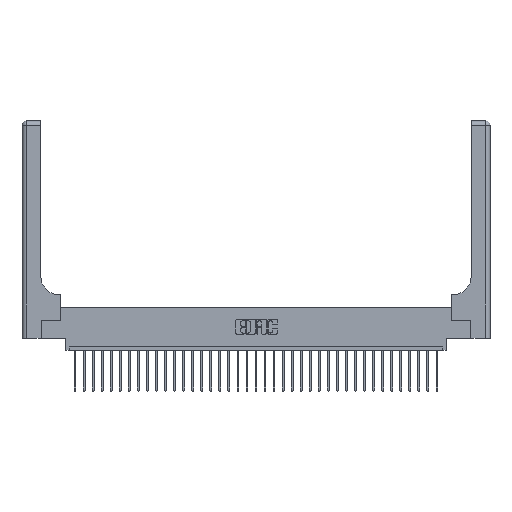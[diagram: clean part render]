
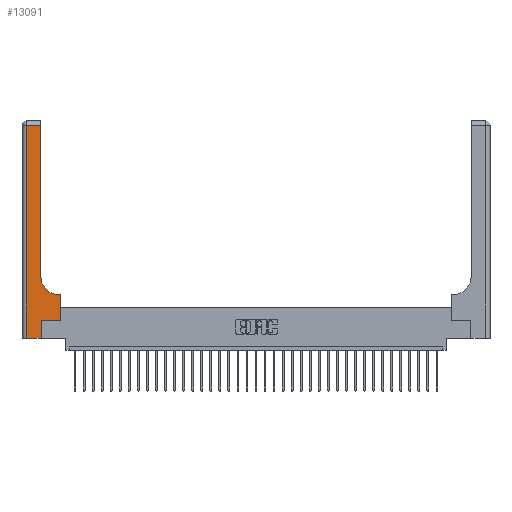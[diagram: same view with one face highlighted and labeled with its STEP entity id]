
A CAD part, top view. The second image highlights one B-rep face of the part: STEP entity #13091.
In plain terms, the highlighted planar face has unit normal (0, 0, 1).
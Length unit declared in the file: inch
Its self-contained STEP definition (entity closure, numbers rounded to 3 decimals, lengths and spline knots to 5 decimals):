
#125 = DIRECTION ( 'NONE',  ( 1., 0., 0. ) ) ;
#1809 = CARTESIAN_POINT ( 'NONE',  ( 0.06, 0., 0.37 ) ) ;
#1960 = DIRECTION ( 'NONE',  ( -1., 0., 0. ) ) ;
#2320 = CARTESIAN_POINT ( 'NONE',  ( 0.51, 0.85, 0.37 ) ) ;
#2383 = CARTESIAN_POINT ( 'NONE',  ( 0.528, 0.25, 0.37 ) ) ;
#2593 = VECTOR ( 'NONE', #26936, 39.37008 ) ;
#3012 = FACE_OUTER_BOUND ( 'NONE', #13031, .T. ) ;
#3409 = EDGE_CURVE ( 'NONE', #23320, #7445, #30415, .T. ) ;
#4195 = LINE ( 'NONE', #17015, #16470 ) ;
#4759 = DIRECTION ( 'NONE',  ( 0., 0., -1. ) ) ;
#5008 = AXIS2_PLACEMENT_3D ( 'NONE', #2320, #4759, #28682 ) ;
#5239 = CARTESIAN_POINT ( 'NONE',  ( 0.528, 0.6, 0.37 ) ) ;
#5479 = EDGE_CURVE ( 'NONE', #10834, #18629, #26133, .T. ) ;
#5733 = CARTESIAN_POINT ( 'NONE',  ( 0.265, 0.25, 0.37 ) ) ;
#6533 = VERTEX_POINT ( 'NONE', #14862 ) ;
#6943 = VECTOR ( 'NONE', #17289, 39.37008 ) ;
#7005 = PLANE ( 'NONE',  #17234 ) ;
#7445 = VERTEX_POINT ( 'NONE', #5239 ) ;
#8553 = CARTESIAN_POINT ( 'NONE',  ( 0., 2.94, 0.37 ) ) ;
#9556 = VECTOR ( 'NONE', #28426, 39.37008 ) ;
#9853 = CARTESIAN_POINT ( 'NONE',  ( 0.26, 0.85, 0.37 ) ) ;
#10433 = CARTESIAN_POINT ( 'NONE',  ( 0.265, 0., 0.37 ) ) ;
#10435 = CARTESIAN_POINT ( 'NONE',  ( 0.265, 0.25, 0.37 ) ) ;
#10453 = LINE ( 'NONE', #10433, #2593 ) ;
#10834 = VERTEX_POINT ( 'NONE', #20953 ) ;
#11054 = VECTOR ( 'NONE', #26046, 39.37008 ) ;
#11936 = CARTESIAN_POINT ( 'NONE',  ( 0., 3., 0.37 ) ) ;
#11959 = CARTESIAN_POINT ( 'NONE',  ( 0.26, 3., 0.37 ) ) ;
#11973 = EDGE_CURVE ( 'NONE', #17200, #23320, #24290, .T. ) ;
#12100 = ORIENTED_EDGE ( 'NONE', *, *, #3409, .T. ) ;
#12642 = CARTESIAN_POINT ( 'NONE',  ( 0.06, 3., 0.37 ) ) ;
#13011 = ORIENTED_EDGE ( 'NONE', *, *, #28578, .T. ) ;
#13031 = EDGE_LOOP ( 'NONE', ( #13040, #22648, #26580, #20272, #13011, #15381, #12100, #23800, #23835 ) ) ;
#13040 = ORIENTED_EDGE ( 'NONE', *, *, #22293, .T. ) ;
#13091 = ADVANCED_FACE ( 'NONE', ( #3012 ), #7005, .F. ) ;
#13892 = CARTESIAN_POINT ( 'NONE',  ( 0.265, 0., 0.37 ) ) ;
#14809 = LINE ( 'NONE', #12642, #6943 ) ;
#14862 = CARTESIAN_POINT ( 'NONE',  ( 0.06, 2.94, 0.37 ) ) ;
#15381 = ORIENTED_EDGE ( 'NONE', *, *, #11973, .T. ) ;
#16470 = VECTOR ( 'NONE', #125, 39.37008 ) ;
#16559 = VECTOR ( 'NONE', #24333, 39.37008 ) ;
#17015 = CARTESIAN_POINT ( 'NONE',  ( 0., 0., 0.37 ) ) ;
#17032 = LINE ( 'NONE', #8553, #9556 ) ;
#17200 = VERTEX_POINT ( 'NONE', #10435 ) ;
#17234 = AXIS2_PLACEMENT_3D ( 'NONE', #11936, #28240, #1960 ) ;
#17289 = DIRECTION ( 'NONE',  ( 0., -1., 0. ) ) ;
#18629 = VERTEX_POINT ( 'NONE', #9853 ) ;
#20165 = EDGE_CURVE ( 'NONE', #7445, #10834, #25524, .T. ) ;
#20272 = ORIENTED_EDGE ( 'NONE', *, *, #22171, .T. ) ;
#20328 = VERTEX_POINT ( 'NONE', #13892 ) ;
#20953 = CARTESIAN_POINT ( 'NONE',  ( 0.51, 0.6, 0.37 ) ) ;
#22171 = EDGE_CURVE ( 'NONE', #27463, #20328, #4195, .T. ) ;
#22293 = EDGE_CURVE ( 'NONE', #18629, #30675, #28382, .T. ) ;
#22648 = ORIENTED_EDGE ( 'NONE', *, *, #24097, .T. ) ;
#23193 = VECTOR ( 'NONE', #26748, 39.37008 ) ;
#23320 = VERTEX_POINT ( 'NONE', #2383 ) ;
#23667 = CARTESIAN_POINT ( 'NONE',  ( 0.528, 0.25, 0.37 ) ) ;
#23800 = ORIENTED_EDGE ( 'NONE', *, *, #20165, .T. ) ;
#23835 = ORIENTED_EDGE ( 'NONE', *, *, #5479, .T. ) ;
#24097 = EDGE_CURVE ( 'NONE', #30675, #6533, #17032, .T. ) ;
#24290 = LINE ( 'NONE', #5733, #23193 ) ;
#24333 = DIRECTION ( 'NONE',  ( -1., 0., 0. ) ) ;
#25524 = LINE ( 'NONE', #28798, #16559 ) ;
#26046 = DIRECTION ( 'NONE',  ( 0., 1., 0. ) ) ;
#26133 = CIRCLE ( 'NONE', #5008, 0.25 ) ;
#26334 = CARTESIAN_POINT ( 'NONE',  ( 0.26, 2.94, 0.37 ) ) ;
#26580 = ORIENTED_EDGE ( 'NONE', *, *, #30844, .T. ) ;
#26748 = DIRECTION ( 'NONE',  ( 1., 0., 0. ) ) ;
#26888 = VECTOR ( 'NONE', #28781, 39.37008 ) ;
#26936 = DIRECTION ( 'NONE',  ( 0., 1., 0. ) ) ;
#27463 = VERTEX_POINT ( 'NONE', #1809 ) ;
#28240 = DIRECTION ( 'NONE',  ( 0., 0., -1. ) ) ;
#28382 = LINE ( 'NONE', #11959, #26888 ) ;
#28426 = DIRECTION ( 'NONE',  ( -1., 0., 0. ) ) ;
#28578 = EDGE_CURVE ( 'NONE', #20328, #17200, #10453, .T. ) ;
#28682 = DIRECTION ( 'NONE',  ( 1., 0., 0. ) ) ;
#28781 = DIRECTION ( 'NONE',  ( 0., 1., 0. ) ) ;
#28798 = CARTESIAN_POINT ( 'NONE',  ( 0.26, 0.6, 0.37 ) ) ;
#30415 = LINE ( 'NONE', #23667, #11054 ) ;
#30675 = VERTEX_POINT ( 'NONE', #26334 ) ;
#30844 = EDGE_CURVE ( 'NONE', #6533, #27463, #14809, .T. ) ;
